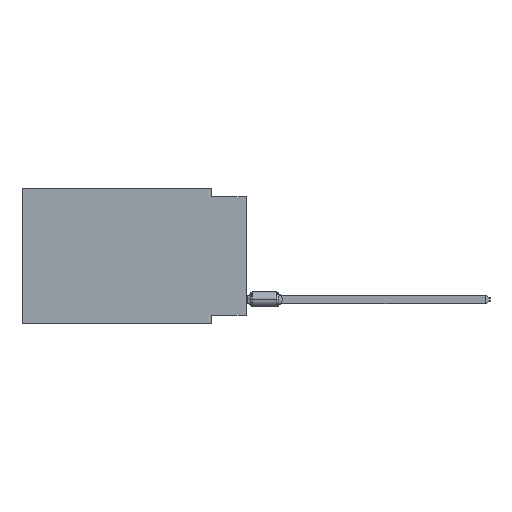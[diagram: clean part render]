
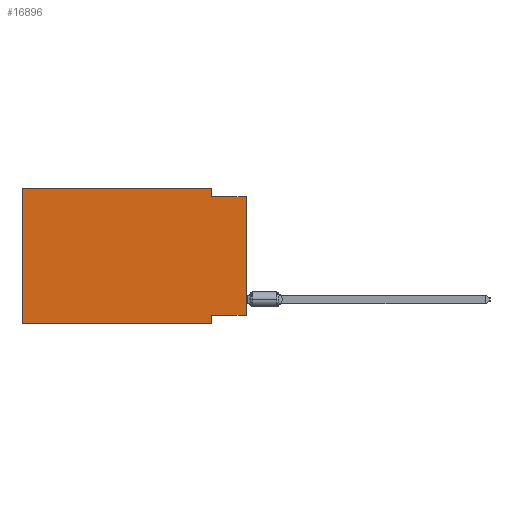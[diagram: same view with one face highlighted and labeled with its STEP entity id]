
A CAD part, left-side view. The second image highlights one B-rep face of the part: STEP entity #16896.
In plain terms, the highlighted planar face has unit normal (-1, 0, 0).
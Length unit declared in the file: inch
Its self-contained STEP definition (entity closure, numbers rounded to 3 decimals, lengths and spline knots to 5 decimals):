
#1454 = CARTESIAN_POINT ( 'NONE',  ( 0., 0.645, 0. ) ) ;
#1745 = EDGE_LOOP ( 'NONE', ( #41245, #5220, #3436, #2092, #9405, #13880, #5299, #25016 ) ) ;
#2092 = ORIENTED_EDGE ( 'NONE', *, *, #19340, .F. ) ;
#2768 = VECTOR ( 'NONE', #22730, 39.37008 ) ;
#3436 = ORIENTED_EDGE ( 'NONE', *, *, #82326, .F. ) ;
#3691 = DIRECTION ( 'NONE',  ( 0., -1., 0. ) ) ;
#4950 = EDGE_CURVE ( 'NONE', #38597, #33361, #14371, .T. ) ;
#5220 = ORIENTED_EDGE ( 'NONE', *, *, #7180, .F. ) ;
#5299 = ORIENTED_EDGE ( 'NONE', *, *, #4950, .F. ) ;
#6427 = LINE ( 'NONE', #43610, #79754 ) ;
#7180 = EDGE_CURVE ( 'NONE', #19074, #10681, #67186, .T. ) ;
#9405 = ORIENTED_EDGE ( 'NONE', *, *, #35777, .F. ) ;
#10284 = LINE ( 'NONE', #29508, #22405 ) ;
#10681 = VERTEX_POINT ( 'NONE', #68722 ) ;
#13593 = LINE ( 'NONE', #1454, #45714 ) ;
#13880 = ORIENTED_EDGE ( 'NONE', *, *, #57578, .T. ) ;
#14297 = DIRECTION ( 'NONE',  ( 1., 0., 0. ) ) ;
#14371 = LINE ( 'NONE', #77040, #39267 ) ;
#16896 = ADVANCED_FACE ( 'NONE', ( #40605 ), #39357, .F. ) ;
#17140 = VERTEX_POINT ( 'NONE', #55990 ) ;
#19074 = VERTEX_POINT ( 'NONE', #60035 ) ;
#19340 = EDGE_CURVE ( 'NONE', #17140, #79182, #13593, .T. ) ;
#19830 = DIRECTION ( 'NONE',  ( 0., 0., -1. ) ) ;
#22405 = VECTOR ( 'NONE', #68323, 39.37008 ) ;
#22730 = DIRECTION ( 'NONE',  ( 0., -1., 0. ) ) ;
#25016 = ORIENTED_EDGE ( 'NONE', *, *, #50252, .F. ) ;
#26969 = DIRECTION ( 'NONE',  ( 0., -1., 0. ) ) ;
#27416 = EDGE_CURVE ( 'NONE', #67596, #10681, #6427, .T. ) ;
#29508 = CARTESIAN_POINT ( 'NONE',  ( 0., 0.645, 0. ) ) ;
#32269 = CARTESIAN_POINT ( 'NONE',  ( 0., 0.1, 0. ) ) ;
#33361 = VERTEX_POINT ( 'NONE', #64417 ) ;
#35777 = EDGE_CURVE ( 'NONE', #79559, #17140, #10284, .T. ) ;
#38597 = VERTEX_POINT ( 'NONE', #59625 ) ;
#39267 = VECTOR ( 'NONE', #19830, 39.37008 ) ;
#39357 = PLANE ( 'NONE',  #73453 ) ;
#40605 = FACE_OUTER_BOUND ( 'NONE', #1745, .T. ) ;
#40634 = VECTOR ( 'NONE', #3691, 39.37008 ) ;
#41245 = ORIENTED_EDGE ( 'NONE', *, *, #27416, .T. ) ;
#43335 = VECTOR ( 'NONE', #49528, 39.37008 ) ;
#43610 = CARTESIAN_POINT ( 'NONE',  ( 0., 0., 0. ) ) ;
#43987 = LINE ( 'NONE', #32269, #65118 ) ;
#44096 = CARTESIAN_POINT ( 'NONE',  ( 0., 0., -0.365 ) ) ;
#45230 = CARTESIAN_POINT ( 'NONE',  ( 0., 0.645, 0. ) ) ;
#45714 = VECTOR ( 'NONE', #26969, 39.37008 ) ;
#48799 = CARTESIAN_POINT ( 'NONE',  ( 0., 0., -0.025 ) ) ;
#49528 = DIRECTION ( 'NONE',  ( 0., 1., 0. ) ) ;
#50252 = EDGE_CURVE ( 'NONE', #67596, #38597, #68738, .T. ) ;
#54104 = CARTESIAN_POINT ( 'NONE',  ( 0., 0.645, -0.39 ) ) ;
#55990 = CARTESIAN_POINT ( 'NONE',  ( 0., 0.645, 0. ) ) ;
#56243 = CARTESIAN_POINT ( 'NONE',  ( 0., 0.1, 0. ) ) ;
#57578 = EDGE_CURVE ( 'NONE', #79559, #33361, #72855, .T. ) ;
#59625 = CARTESIAN_POINT ( 'NONE',  ( 0., 0.1, -0.365 ) ) ;
#60035 = CARTESIAN_POINT ( 'NONE',  ( 0., 0.1, -0.025 ) ) ;
#64417 = CARTESIAN_POINT ( 'NONE',  ( 0., 0.1, -0.39 ) ) ;
#65118 = VECTOR ( 'NONE', #82006, 39.37008 ) ;
#67186 = LINE ( 'NONE', #48799, #40634 ) ;
#67596 = VERTEX_POINT ( 'NONE', #80401 ) ;
#68323 = DIRECTION ( 'NONE',  ( 0., 0., 1. ) ) ;
#68722 = CARTESIAN_POINT ( 'NONE',  ( 0., 0., -0.025 ) ) ;
#68738 = LINE ( 'NONE', #44096, #43335 ) ;
#72855 = LINE ( 'NONE', #73270, #2768 ) ;
#73270 = CARTESIAN_POINT ( 'NONE',  ( 0., 0.645, -0.39 ) ) ;
#73453 = AXIS2_PLACEMENT_3D ( 'NONE', #45230, #14297, #77380 ) ;
#77040 = CARTESIAN_POINT ( 'NONE',  ( 0., 0.1, -0.39 ) ) ;
#77380 = DIRECTION ( 'NONE',  ( 0., 0., -1. ) ) ;
#79182 = VERTEX_POINT ( 'NONE', #56243 ) ;
#79559 = VERTEX_POINT ( 'NONE', #54104 ) ;
#79754 = VECTOR ( 'NONE', #82047, 39.37008 ) ;
#80401 = CARTESIAN_POINT ( 'NONE',  ( 0., 0., -0.365 ) ) ;
#82006 = DIRECTION ( 'NONE',  ( 0., 0., -1. ) ) ;
#82047 = DIRECTION ( 'NONE',  ( 0., 0., 1. ) ) ;
#82326 = EDGE_CURVE ( 'NONE', #79182, #19074, #43987, .T. ) ;
